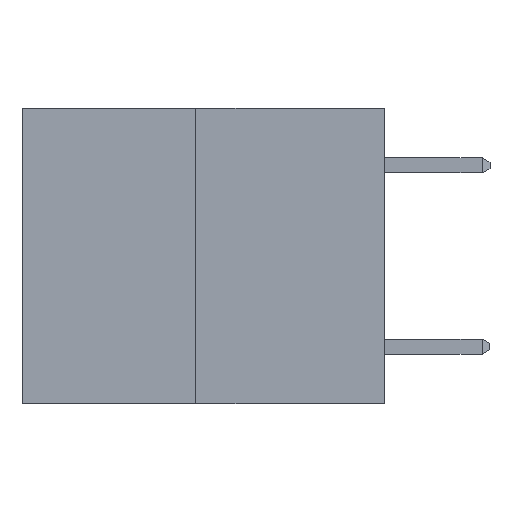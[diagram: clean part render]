
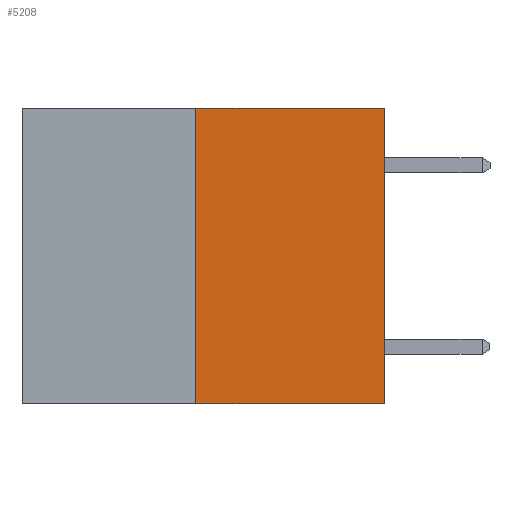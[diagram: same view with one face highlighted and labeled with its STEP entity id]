
A CAD part, left-side view. The second image highlights one B-rep face of the part: STEP entity #5208.
In plain terms, the highlighted planar face has unit normal (-1, 0, 0).
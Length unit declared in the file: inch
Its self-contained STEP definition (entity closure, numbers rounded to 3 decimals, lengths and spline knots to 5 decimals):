
#100 = DIRECTION ( 'NONE',  ( 0., 0., 1. ) ) ;
#658 = VERTEX_POINT ( 'NONE', #12875 ) ;
#1204 = VECTOR ( 'NONE', #4779, 39.37008 ) ;
#1593 = ORIENTED_EDGE ( 'NONE', *, *, #4431, .F. ) ;
#1973 = VECTOR ( 'NONE', #7941, 39.37008 ) ;
#2307 = ORIENTED_EDGE ( 'NONE', *, *, #12252, .F. ) ;
#2986 = AXIS2_PLACEMENT_3D ( 'NONE', #12379, #6383, #11497 ) ;
#3162 = VERTEX_POINT ( 'NONE', #12989 ) ;
#3747 = ORIENTED_EDGE ( 'NONE', *, *, #5201, .T. ) ;
#4085 = LINE ( 'NONE', #7748, #1973 ) ;
#4431 = EDGE_CURVE ( 'NONE', #3162, #4691, #9425, .T. ) ;
#4667 = LINE ( 'NONE', #12749, #6582 ) ;
#4691 = VERTEX_POINT ( 'NONE', #4811 ) ;
#4779 = DIRECTION ( 'NONE',  ( 0., -1., 0. ) ) ;
#4811 = CARTESIAN_POINT ( 'NONE',  ( 0., 0., 0. ) ) ;
#5105 = VERTEX_POINT ( 'NONE', #6267 ) ;
#5201 = EDGE_CURVE ( 'NONE', #5105, #4691, #13340, .T. ) ;
#5208 = ADVANCED_FACE ( 'NONE', ( #11712 ), #10406, .F. ) ;
#5605 = EDGE_CURVE ( 'NONE', #658, #5105, #4667, .T. ) ;
#6267 = CARTESIAN_POINT ( 'NONE',  ( 0., 0., -0.49 ) ) ;
#6383 = DIRECTION ( 'NONE',  ( 1., 0., 0. ) ) ;
#6582 = VECTOR ( 'NONE', #6675, 39.37008 ) ;
#6675 = DIRECTION ( 'NONE',  ( 0., -1., 0. ) ) ;
#7748 = CARTESIAN_POINT ( 'NONE',  ( 0., 0.312, -0.49 ) ) ;
#7941 = DIRECTION ( 'NONE',  ( 0., 0., 1. ) ) ;
#8220 = VECTOR ( 'NONE', #100, 39.37008 ) ;
#8944 = EDGE_LOOP ( 'NONE', ( #2307, #11099, #3747, #1593 ) ) ;
#9425 = LINE ( 'NONE', #12923, #1204 ) ;
#10329 = CARTESIAN_POINT ( 'NONE',  ( 0., 0., 0. ) ) ;
#10406 = PLANE ( 'NONE',  #2986 ) ;
#11099 = ORIENTED_EDGE ( 'NONE', *, *, #5605, .T. ) ;
#11497 = DIRECTION ( 'NONE',  ( 0., 0., -1. ) ) ;
#11712 = FACE_OUTER_BOUND ( 'NONE', #8944, .T. ) ;
#12252 = EDGE_CURVE ( 'NONE', #658, #3162, #4085, .T. ) ;
#12379 = CARTESIAN_POINT ( 'NONE',  ( 0., 0.6, 0. ) ) ;
#12749 = CARTESIAN_POINT ( 'NONE',  ( 0., 0.6, -0.49 ) ) ;
#12875 = CARTESIAN_POINT ( 'NONE',  ( 0., 0.312, -0.49 ) ) ;
#12923 = CARTESIAN_POINT ( 'NONE',  ( 0., 0.6, 0. ) ) ;
#12989 = CARTESIAN_POINT ( 'NONE',  ( 0., 0.312, 0. ) ) ;
#13340 = LINE ( 'NONE', #10329, #8220 ) ;
